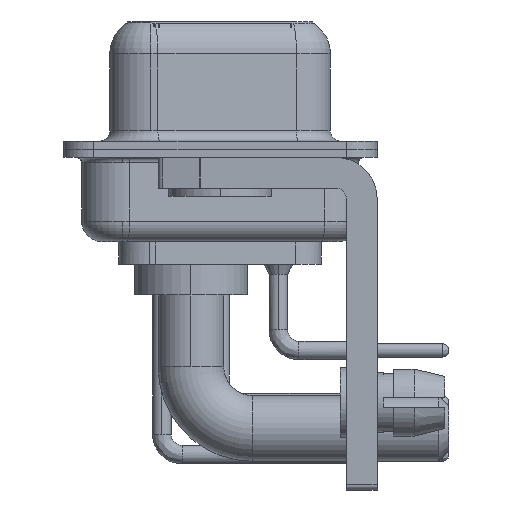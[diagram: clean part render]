
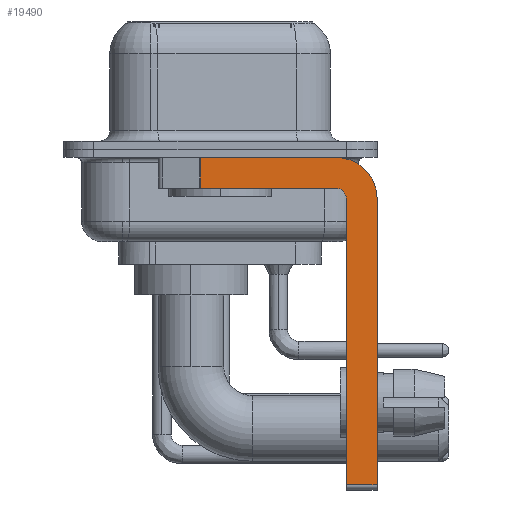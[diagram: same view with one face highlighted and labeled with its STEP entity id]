
A CAD part, left-side view. The second image highlights one B-rep face of the part: STEP entity #19490.
In plain terms, the highlighted planar face has unit normal (-1, 0, 0).
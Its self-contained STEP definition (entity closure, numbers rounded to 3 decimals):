
#188 = LINE ( 'NONE', #21728, #14145 ) ;
#281 = CARTESIAN_POINT ( 'NONE',  ( -2.9, -5.65, -2.4 ) ) ;
#1585 = CARTESIAN_POINT ( 'NONE',  ( -2.9, -5.65, -16.35 ) ) ;
#1603 = DIRECTION ( 'NONE',  ( 0., 0., 1. ) ) ;
#2236 = AXIS2_PLACEMENT_3D ( 'NONE', #25819, #33931, #1603 ) ;
#2246 = DIRECTION ( 'NONE',  ( 0., 0., -1. ) ) ;
#2600 = FACE_OUTER_BOUND ( 'NONE', #21773, .T. ) ;
#2723 = VERTEX_POINT ( 'NONE', #31370 ) ;
#3009 = VECTOR ( 'NONE', #34495, 1000. ) ;
#6339 = CIRCLE ( 'NONE', #11983, 2. ) ;
#7058 = LINE ( 'NONE', #1585, #31869 ) ;
#7638 = CARTESIAN_POINT ( 'NONE',  ( -2.9, -5.65, -1.9 ) ) ;
#9049 = VERTEX_POINT ( 'NONE', #24311 ) ;
#9263 = ORIENTED_EDGE ( 'NONE', *, *, #29461, .F. ) ;
#10142 = CARTESIAN_POINT ( 'NONE',  ( -2.9, 3., -0.4 ) ) ;
#10198 = CARTESIAN_POINT ( 'NONE',  ( -2.9, -5.65, -2.4 ) ) ;
#10595 = CARTESIAN_POINT ( 'NONE',  ( -2.9, -7.65, -2.4 ) ) ;
#10618 = EDGE_CURVE ( 'NONE', #21896, #2723, #23049, .T. ) ;
#10730 = CARTESIAN_POINT ( 'NONE',  ( -2.9, 0.978, -1.9 ) ) ;
#10909 = DIRECTION ( 'NONE',  ( 1., 0., 0. ) ) ;
#11482 = CARTESIAN_POINT ( 'NONE',  ( -2.9, 0.978, -0.4 ) ) ;
#11688 = EDGE_CURVE ( 'NONE', #34289, #18486, #21522, .T. ) ;
#11983 = AXIS2_PLACEMENT_3D ( 'NONE', #10198, #10909, #2246 ) ;
#12277 = LINE ( 'NONE', #33827, #25707 ) ;
#13431 = ORIENTED_EDGE ( 'NONE', *, *, #27658, .F. ) ;
#13465 = VECTOR ( 'NONE', #20836, 1000. ) ;
#13596 = EDGE_CURVE ( 'NONE', #21896, #29108, #188, .T. ) ;
#14079 = CIRCLE ( 'NONE', #2236, 0.5 ) ;
#14145 = VECTOR ( 'NONE', #22257, 1000. ) ;
#14491 = AXIS2_PLACEMENT_3D ( 'NONE', #281, #19199, #32279 ) ;
#15042 = ORIENTED_EDGE ( 'NONE', *, *, #22994, .F. ) ;
#15848 = PLANE ( 'NONE',  #14491 ) ;
#16514 = EDGE_CURVE ( 'NONE', #2723, #34289, #6339, .T. ) ;
#17317 = EDGE_CURVE ( 'NONE', #19038, #18486, #7058, .T. ) ;
#18426 = LINE ( 'NONE', #7638, #3009 ) ;
#18486 = VERTEX_POINT ( 'NONE', #34691 ) ;
#19038 = VERTEX_POINT ( 'NONE', #26743 ) ;
#19199 = DIRECTION ( 'NONE',  ( 1., 0., 0. ) ) ;
#19490 = ADVANCED_FACE ( 'NONE', ( #2600 ), #15848, .F. ) ;
#20836 = DIRECTION ( 'NONE',  ( 0., 0., -1. ) ) ;
#20928 = DIRECTION ( 'NONE',  ( 0., -1., 0. ) ) ;
#21522 = LINE ( 'NONE', #34240, #13465 ) ;
#21728 = CARTESIAN_POINT ( 'NONE',  ( -2.9, 0.978, -1.9 ) ) ;
#21773 = EDGE_LOOP ( 'NONE', ( #33056, #29892, #13431, #15042, #9263, #28822, #22795, #25609 ) ) ;
#21896 = VERTEX_POINT ( 'NONE', #11482 ) ;
#22257 = DIRECTION ( 'NONE',  ( 0., 0., -1. ) ) ;
#22795 = ORIENTED_EDGE ( 'NONE', *, *, #11688, .F. ) ;
#22994 = EDGE_CURVE ( 'NONE', #9049, #34057, #14079, .T. ) ;
#23049 = LINE ( 'NONE', #10142, #33110 ) ;
#24311 = CARTESIAN_POINT ( 'NONE',  ( -2.9, -6.15, -2.4 ) ) ;
#24936 = CARTESIAN_POINT ( 'NONE',  ( -2.9, -5.65, -1.9 ) ) ;
#25609 = ORIENTED_EDGE ( 'NONE', *, *, #16514, .F. ) ;
#25707 = VECTOR ( 'NONE', #31199, 1000. ) ;
#25819 = CARTESIAN_POINT ( 'NONE',  ( -2.9, -5.65, -2.4 ) ) ;
#26743 = CARTESIAN_POINT ( 'NONE',  ( -2.9, -6.15, -16.35 ) ) ;
#27658 = EDGE_CURVE ( 'NONE', #34057, #29108, #18426, .T. ) ;
#28822 = ORIENTED_EDGE ( 'NONE', *, *, #17317, .T. ) ;
#29108 = VERTEX_POINT ( 'NONE', #10730 ) ;
#29461 = EDGE_CURVE ( 'NONE', #19038, #9049, #12277, .T. ) ;
#29892 = ORIENTED_EDGE ( 'NONE', *, *, #13596, .T. ) ;
#31199 = DIRECTION ( 'NONE',  ( 0., 0., 1. ) ) ;
#31370 = CARTESIAN_POINT ( 'NONE',  ( -2.9, -5.65, -0.4 ) ) ;
#31788 = DIRECTION ( 'NONE',  ( 0., -1., 0. ) ) ;
#31869 = VECTOR ( 'NONE', #31788, 1000. ) ;
#32279 = DIRECTION ( 'NONE',  ( 0., 0., -1. ) ) ;
#33056 = ORIENTED_EDGE ( 'NONE', *, *, #10618, .F. ) ;
#33110 = VECTOR ( 'NONE', #20928, 1000. ) ;
#33827 = CARTESIAN_POINT ( 'NONE',  ( -2.9, -6.15, -16.6 ) ) ;
#33931 = DIRECTION ( 'NONE',  ( -1., 0., 0. ) ) ;
#34057 = VERTEX_POINT ( 'NONE', #24936 ) ;
#34240 = CARTESIAN_POINT ( 'NONE',  ( -2.9, -7.65, -2.4 ) ) ;
#34289 = VERTEX_POINT ( 'NONE', #10595 ) ;
#34495 = DIRECTION ( 'NONE',  ( 0., 1., 0. ) ) ;
#34691 = CARTESIAN_POINT ( 'NONE',  ( -2.9, -7.65, -16.35 ) ) ;
